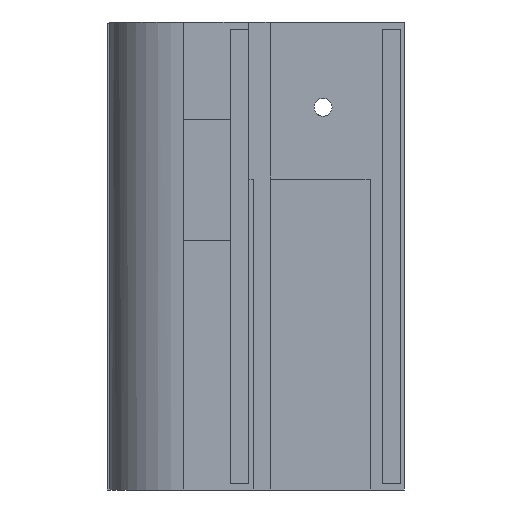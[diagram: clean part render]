
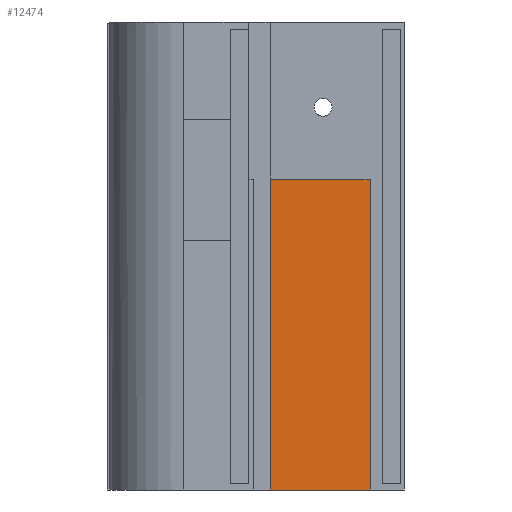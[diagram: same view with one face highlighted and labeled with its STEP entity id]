
A CAD part, left-side view. The second image highlights one B-rep face of the part: STEP entity #12474.
In plain terms, the highlighted planar face has unit normal (-1, 0, 0).
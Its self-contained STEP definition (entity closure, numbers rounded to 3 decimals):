
#2883 = PLANE('',#2884);
#2884 = AXIS2_PLACEMENT_3D('',#2885,#2886,#2887);
#2885 = CARTESIAN_POINT('',(-13.,45.608,-1.));
#2886 = DIRECTION('',(1.,0.,0.));
#2887 = DIRECTION('',(0.,-1.,0.));
#2909 = PLANE('',#2910);
#2910 = AXIS2_PLACEMENT_3D('',#2911,#2912,#2913);
#2911 = CARTESIAN_POINT('',(-13.,-10.668,-1.));
#2912 = DIRECTION('',(-1.,0.,0.));
#2913 = DIRECTION('',(0.,1.,0.));
#7124 = VERTEX_POINT('',#7125);
#7125 = CARTESIAN_POINT('',(-13.,-5.,-1.));
#7171 = VERTEX_POINT('',#7172);
#7172 = CARTESIAN_POINT('',(-13.,11.467,50.19));
#7192 = EDGE_CURVE('',#7193,#7171,#7195,.T.);
#7193 = VERTEX_POINT('',#7194);
#7194 = CARTESIAN_POINT('',(-13.,-5.,50.19));
#7195 = SURFACE_CURVE('',#7196,(#7200,#7207),.PCURVE_S1.);
#7196 = LINE('',#7197,#7198);
#7197 = CARTESIAN_POINT('',(-13.,26.544,50.19));
#7198 = VECTOR('',#7199,1.);
#7199 = DIRECTION('',(0.,1.,0.));
#7200 = PCURVE('',#2909,#7201);
#7201 = DEFINITIONAL_REPRESENTATION('',(#7202),#7206);
#7202 = LINE('',#7203,#7204);
#7203 = CARTESIAN_POINT('',(37.212,-51.19));
#7204 = VECTOR('',#7205,1.);
#7205 = DIRECTION('',(1.,0.));
#7206 = ( GEOMETRIC_REPRESENTATION_CONTEXT(2) 
PARAMETRIC_REPRESENTATION_CONTEXT() REPRESENTATION_CONTEXT('2D SPACE',''
  ) );
#7207 = PCURVE('',#7208,#7213);
#7208 = PLANE('',#7209);
#7209 = AXIS2_PLACEMENT_3D('',#7210,#7211,#7212);
#7210 = CARTESIAN_POINT('',(-13.,39.89,-1.));
#7211 = DIRECTION('',(1.,0.,0.));
#7212 = DIRECTION('',(0.,-1.,0.));
#7213 = DEFINITIONAL_REPRESENTATION('',(#7214),#7217);
#7214 = B_SPLINE_CURVE_WITH_KNOTS('',1,(#7215,#7216),.UNSPECIFIED.,.F.,
  .F.,(2,2),(-36.033,17.835),.PIECEWISE_BEZIER_KNOTS.);
#7215 = CARTESIAN_POINT('',(49.379,-51.19));
#7216 = CARTESIAN_POINT('',(-4.489,-51.19));
#7217 = ( GEOMETRIC_REPRESENTATION_CONTEXT(2) 
PARAMETRIC_REPRESENTATION_CONTEXT() REPRESENTATION_CONTEXT('2D SPACE',''
  ) );
#7219 = EDGE_CURVE('',#7124,#7193,#7220,.T.);
#7220 = SURFACE_CURVE('',#7221,(#7225,#7232),.PCURVE_S1.);
#7221 = LINE('',#7222,#7223);
#7222 = CARTESIAN_POINT('',(-13.,-5.,-1.));
#7223 = VECTOR('',#7224,1.);
#7224 = DIRECTION('',(0.,0.,1.));
#7225 = PCURVE('',#2909,#7226);
#7226 = DEFINITIONAL_REPRESENTATION('',(#7227),#7231);
#7227 = LINE('',#7228,#7229);
#7228 = CARTESIAN_POINT('',(5.668,0.));
#7229 = VECTOR('',#7230,1.);
#7230 = DIRECTION('',(0.,-1.));
#7231 = ( GEOMETRIC_REPRESENTATION_CONTEXT(2) 
PARAMETRIC_REPRESENTATION_CONTEXT() REPRESENTATION_CONTEXT('2D SPACE',''
  ) );
#7232 = PCURVE('',#7208,#7233);
#7233 = DEFINITIONAL_REPRESENTATION('',(#7234),#7238);
#7234 = LINE('',#7235,#7236);
#7235 = CARTESIAN_POINT('',(44.89,0.));
#7236 = VECTOR('',#7237,1.);
#7237 = DIRECTION('',(0.,-1.));
#7238 = ( GEOMETRIC_REPRESENTATION_CONTEXT(2) 
PARAMETRIC_REPRESENTATION_CONTEXT() REPRESENTATION_CONTEXT('2D SPACE',''
  ) );
#7395 = VERTEX_POINT('',#7396);
#7396 = CARTESIAN_POINT('',(-13.,11.467,-1.));
#7594 = EDGE_CURVE('',#7595,#7171,#7597,.T.);
#7595 = VERTEX_POINT('',#7596);
#7596 = CARTESIAN_POINT('',(-13.,11.467,49.82));
#7597 = SURFACE_CURVE('',#7598,(#7602,#7609),.PCURVE_S1.);
#7598 = LINE('',#7599,#7600);
#7599 = CARTESIAN_POINT('',(-13.,11.467,-1.));
#7600 = VECTOR('',#7601,1.);
#7601 = DIRECTION('',(0.,0.,1.));
#7602 = PCURVE('',#2883,#7603);
#7603 = DEFINITIONAL_REPRESENTATION('',(#7604),#7608);
#7604 = LINE('',#7605,#7606);
#7605 = CARTESIAN_POINT('',(34.141,0.));
#7606 = VECTOR('',#7607,1.);
#7607 = DIRECTION('',(0.,-1.));
#7608 = ( GEOMETRIC_REPRESENTATION_CONTEXT(2) 
PARAMETRIC_REPRESENTATION_CONTEXT() REPRESENTATION_CONTEXT('2D SPACE',''
  ) );
#7609 = PCURVE('',#7208,#7610);
#7610 = DEFINITIONAL_REPRESENTATION('',(#7611),#7614);
#7611 = B_SPLINE_CURVE_WITH_KNOTS('',1,(#7612,#7613),.UNSPECIFIED.,.F.,
  .F.,(2,2),(50.702,52.118),.PIECEWISE_BEZIER_KNOTS.);
#7612 = CARTESIAN_POINT('',(28.423,-50.702));
#7613 = CARTESIAN_POINT('',(28.423,-52.118));
#7614 = ( GEOMETRIC_REPRESENTATION_CONTEXT(2) 
PARAMETRIC_REPRESENTATION_CONTEXT() REPRESENTATION_CONTEXT('2D SPACE',''
  ) );
#7616 = EDGE_CURVE('',#7395,#7595,#7617,.T.);
#7617 = SURFACE_CURVE('',#7618,(#7622,#7629),.PCURVE_S1.);
#7618 = LINE('',#7619,#7620);
#7619 = CARTESIAN_POINT('',(-13.,11.467,-1.));
#7620 = VECTOR('',#7621,1.);
#7621 = DIRECTION('',(0.,0.,1.));
#7622 = PCURVE('',#2883,#7623);
#7623 = DEFINITIONAL_REPRESENTATION('',(#7624),#7628);
#7624 = LINE('',#7625,#7626);
#7625 = CARTESIAN_POINT('',(34.141,0.));
#7626 = VECTOR('',#7627,1.);
#7627 = DIRECTION('',(0.,-1.));
#7628 = ( GEOMETRIC_REPRESENTATION_CONTEXT(2) 
PARAMETRIC_REPRESENTATION_CONTEXT() REPRESENTATION_CONTEXT('2D SPACE',''
  ) );
#7629 = PCURVE('',#7208,#7630);
#7630 = DEFINITIONAL_REPRESENTATION('',(#7631),#7634);
#7631 = B_SPLINE_CURVE_WITH_KNOTS('',1,(#7632,#7633),.UNSPECIFIED.,.F.,
  .F.,(2,2),(-5.082,55.902),.PIECEWISE_BEZIER_KNOTS.);
#7632 = CARTESIAN_POINT('',(28.423,5.082));
#7633 = CARTESIAN_POINT('',(28.423,-55.902));
#7634 = ( GEOMETRIC_REPRESENTATION_CONTEXT(2) 
PARAMETRIC_REPRESENTATION_CONTEXT() REPRESENTATION_CONTEXT('2D SPACE',''
  ) );
#12437 = PLANE('',#12438);
#12438 = AXIS2_PLACEMENT_3D('',#12439,#12440,#12441);
#12439 = CARTESIAN_POINT('',(-13.,-5.,-1.));
#12440 = DIRECTION('',(0.,0.,-1.));
#12441 = DIRECTION('',(-1.,0.,0.));
#12474 = ADVANCED_FACE('',(#12475),#7208,.F.);
#12475 = FACE_BOUND('',#12476,.F.);
#12476 = EDGE_LOOP('',(#12477,#12498,#12499,#12500,#12501));
#12477 = ORIENTED_EDGE('',*,*,#12478,.F.);
#12478 = EDGE_CURVE('',#7395,#7124,#12479,.T.);
#12479 = SURFACE_CURVE('',#12480,(#12484,#12491),.PCURVE_S1.);
#12480 = LINE('',#12481,#12482);
#12481 = CARTESIAN_POINT('',(-13.,45.608,-1.));
#12482 = VECTOR('',#12483,1.);
#12483 = DIRECTION('',(0.,-1.,0.));
#12484 = PCURVE('',#7208,#12485);
#12485 = DEFINITIONAL_REPRESENTATION('',(#12486),#12490);
#12486 = LINE('',#12487,#12488);
#12487 = CARTESIAN_POINT('',(-5.718,0.));
#12488 = VECTOR('',#12489,1.);
#12489 = DIRECTION('',(1.,0.));
#12490 = ( GEOMETRIC_REPRESENTATION_CONTEXT(2) 
PARAMETRIC_REPRESENTATION_CONTEXT() REPRESENTATION_CONTEXT('2D SPACE',''
  ) );
#12491 = PCURVE('',#12437,#12492);
#12492 = DEFINITIONAL_REPRESENTATION('',(#12493),#12497);
#12493 = LINE('',#12494,#12495);
#12494 = CARTESIAN_POINT('',(0.,50.608));
#12495 = VECTOR('',#12496,1.);
#12496 = DIRECTION('',(0.,-1.));
#12497 = ( GEOMETRIC_REPRESENTATION_CONTEXT(2) 
PARAMETRIC_REPRESENTATION_CONTEXT() REPRESENTATION_CONTEXT('2D SPACE',''
  ) );
#12498 = ORIENTED_EDGE('',*,*,#7616,.T.);
#12499 = ORIENTED_EDGE('',*,*,#7594,.T.);
#12500 = ORIENTED_EDGE('',*,*,#7192,.F.);
#12501 = ORIENTED_EDGE('',*,*,#7219,.F.);
